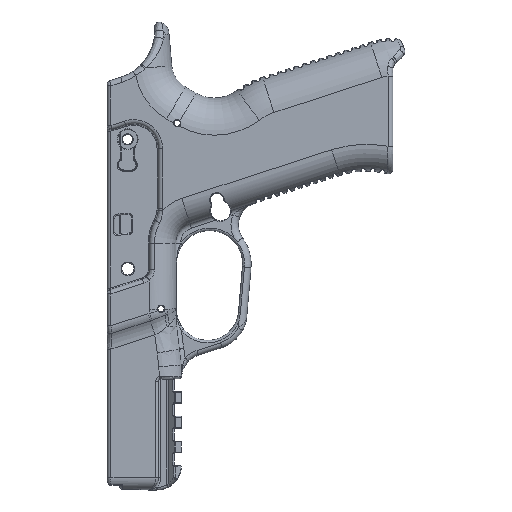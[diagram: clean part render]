
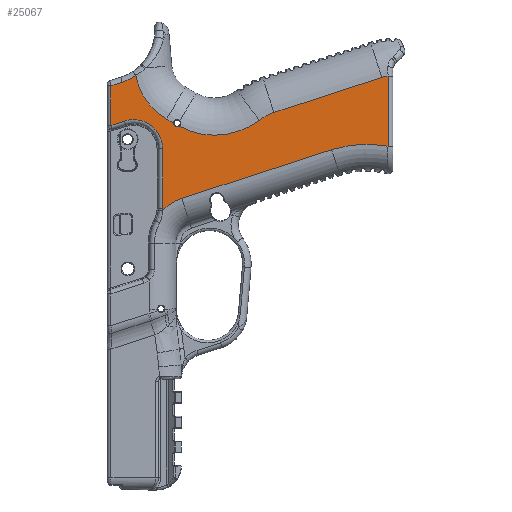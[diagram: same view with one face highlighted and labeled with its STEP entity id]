
A CAD part, left-side view. The second image highlights one B-rep face of the part: STEP entity #25067.
In plain terms, the highlighted planar face has unit normal (-1, 0, 0).
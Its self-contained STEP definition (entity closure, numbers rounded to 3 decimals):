
#246=PLANE('',#27413);
#535=LINE('',#38847,#1671);
#678=LINE('',#45280,#1814);
#984=LINE('',#53656,#2120);
#985=LINE('',#53662,#2121);
#986=LINE('',#53664,#2122);
#987=LINE('',#53666,#2123);
#988=LINE('',#53670,#2124);
#989=LINE('',#53675,#2125);
#1671=VECTOR('',#29705,10.);
#1814=VECTOR('',#30608,10.);
#2120=VECTOR('',#32378,10.);
#2121=VECTOR('',#32383,10.);
#2122=VECTOR('',#32384,10.);
#2123=VECTOR('',#32385,10.);
#2124=VECTOR('',#32388,10.);
#2125=VECTOR('',#32393,10.);
#4097=FACE_OUTER_BOUND('',#5734,.T.);
#5734=EDGE_LOOP('',(#19691,#19692,#19693,#19694,#19695,#19696,#19697,#19698,
#19699,#19700,#19701,#19702,#19703,#19704,#19705,#19706,#19707,#19708,#19709,
#19710));
#7162=CIRCLE('',#26238,20.);
#7449=CIRCLE('',#26915,46.);
#7712=CIRCLE('',#27407,1.44);
#7714=CIRCLE('',#27410,30.);
#7717=CIRCLE('',#27414,26.);
#7718=CIRCLE('',#27415,22.);
#7719=CIRCLE('',#27416,11.75);
#7720=CIRCLE('',#27417,11.75);
#7721=CIRCLE('',#27418,19.);
#7722=CIRCLE('',#27419,13.);
#9006=B_SPLINE_CURVE_WITH_KNOTS('',3,(#53617,#53618,#53619,#53620),
 .UNSPECIFIED.,.F.,.F.,(4,4),(0.244,0.253),
 .UNSPECIFIED.);
#9008=B_SPLINE_CURVE_WITH_KNOTS('',3,(#53641,#53642,#53643,#53644),
 .UNSPECIFIED.,.F.,.F.,(4,4),(0.052,0.062),
 .UNSPECIFIED.);
#9708=VERTEX_POINT('',#37754);
#9709=VERTEX_POINT('',#37756);
#9775=VERTEX_POINT('',#38846);
#10185=VERTEX_POINT('',#45277);
#10186=VERTEX_POINT('',#45279);
#10414=VERTEX_POINT('',#49002);
#10813=VERTEX_POINT('',#53458);
#10817=VERTEX_POINT('',#53496);
#10818=VERTEX_POINT('',#53498);
#10820=VERTEX_POINT('',#53563);
#10824=VERTEX_POINT('',#53655);
#10825=VERTEX_POINT('',#53657);
#10826=VERTEX_POINT('',#53659);
#10827=VERTEX_POINT('',#53661);
#10828=VERTEX_POINT('',#53663);
#10829=VERTEX_POINT('',#53665);
#10830=VERTEX_POINT('',#53667);
#10831=VERTEX_POINT('',#53669);
#10832=VERTEX_POINT('',#53671);
#10833=VERTEX_POINT('',#53674);
#12171=EDGE_CURVE('',#9708,#9709,#7162,.T.);
#12275=EDGE_CURVE('',#9709,#9775,#535,.T.);
#12896=EDGE_CURVE('',#10185,#10186,#678,.T.);
#13259=EDGE_CURVE('',#10414,#10185,#7449,.T.);
#13918=EDGE_CURVE('',#10817,#10818,#7712,.T.);
#13925=EDGE_CURVE('',#10820,#10817,#9006,.T.);
#13927=EDGE_CURVE('',#10818,#10813,#9008,.T.);
#13929=EDGE_CURVE('',#10813,#9708,#7714,.T.);
#13932=EDGE_CURVE('',#10824,#10820,#984,.T.);
#13933=EDGE_CURVE('',#10825,#10824,#7717,.T.);
#13934=EDGE_CURVE('',#10826,#10825,#7718,.T.);
#13935=EDGE_CURVE('',#10827,#10826,#985,.T.);
#13936=EDGE_CURVE('',#10828,#10827,#986,.T.);
#13937=EDGE_CURVE('',#10829,#10828,#987,.T.);
#13938=EDGE_CURVE('',#10830,#10829,#7719,.T.);
#13939=EDGE_CURVE('',#10831,#10830,#988,.T.);
#13940=EDGE_CURVE('',#10832,#10831,#7720,.T.);
#13941=EDGE_CURVE('',#10186,#10832,#7721,.T.);
#13942=EDGE_CURVE('',#10833,#10414,#989,.T.);
#13943=EDGE_CURVE('',#9775,#10833,#7722,.T.);
#19691=ORIENTED_EDGE('',*,*,#13927,.F.);
#19692=ORIENTED_EDGE('',*,*,#13918,.F.);
#19693=ORIENTED_EDGE('',*,*,#13925,.F.);
#19694=ORIENTED_EDGE('',*,*,#13932,.F.);
#19695=ORIENTED_EDGE('',*,*,#13933,.F.);
#19696=ORIENTED_EDGE('',*,*,#13934,.F.);
#19697=ORIENTED_EDGE('',*,*,#13935,.F.);
#19698=ORIENTED_EDGE('',*,*,#13936,.F.);
#19699=ORIENTED_EDGE('',*,*,#13937,.F.);
#19700=ORIENTED_EDGE('',*,*,#13938,.F.);
#19701=ORIENTED_EDGE('',*,*,#13939,.F.);
#19702=ORIENTED_EDGE('',*,*,#13940,.F.);
#19703=ORIENTED_EDGE('',*,*,#13941,.F.);
#19704=ORIENTED_EDGE('',*,*,#12896,.F.);
#19705=ORIENTED_EDGE('',*,*,#13259,.F.);
#19706=ORIENTED_EDGE('',*,*,#13942,.F.);
#19707=ORIENTED_EDGE('',*,*,#13943,.F.);
#19708=ORIENTED_EDGE('',*,*,#12275,.F.);
#19709=ORIENTED_EDGE('',*,*,#12171,.F.);
#19710=ORIENTED_EDGE('',*,*,#13929,.F.);
#25067=ADVANCED_FACE('',(#4097),#246,.F.);
#26238=AXIS2_PLACEMENT_3D('',#37757,#29557,#29558);
#26915=AXIS2_PLACEMENT_3D('',#49010,#31153,#31154);
#27407=AXIS2_PLACEMENT_3D('',#53499,#32362,#32363);
#27410=AXIS2_PLACEMENT_3D('',#53650,#32370,#32371);
#27413=AXIS2_PLACEMENT_3D('',#53654,#32376,#32377);
#27414=AXIS2_PLACEMENT_3D('',#53658,#32379,#32380);
#27415=AXIS2_PLACEMENT_3D('',#53660,#32381,#32382);
#27416=AXIS2_PLACEMENT_3D('',#53668,#32386,#32387);
#27417=AXIS2_PLACEMENT_3D('',#53672,#32389,#32390);
#27418=AXIS2_PLACEMENT_3D('',#53673,#32391,#32392);
#27419=AXIS2_PLACEMENT_3D('',#53676,#32394,#32395);
#29557=DIRECTION('center_axis',(1.,0.,0.));
#29558=DIRECTION('ref_axis',(0.,0.463,0.886));
#29705=DIRECTION('',(0.,-0.951,0.309));
#30608=DIRECTION('',(0.,0.951,-0.309));
#31153=DIRECTION('center_axis',(-1.,0.,0.));
#31154=DIRECTION('ref_axis',(0.,-0.012,1.));
#32362=DIRECTION('center_axis',(-1.,0.,0.));
#32363=DIRECTION('ref_axis',(0.,0.,-1.));
#32370=DIRECTION('center_axis',(-1.,0.,0.));
#32371=DIRECTION('ref_axis',(0.,-0.062,-0.998));
#32376=DIRECTION('center_axis',(1.,0.,0.));
#32377=DIRECTION('ref_axis',(0.,0.,-1.));
#32378=DIRECTION('',(0.,-0.866,-0.5));
#32379=DIRECTION('center_axis',(-1.,0.,0.));
#32380=DIRECTION('ref_axis',(0.,0.843,-0.537));
#32381=DIRECTION('center_axis',(-1.,0.,0.));
#32382=DIRECTION('ref_axis',(0.,-0.459,-0.889));
#32383=DIRECTION('',(0.,-0.951,0.309));
#32384=DIRECTION('',(0.,0.,1.));
#32385=DIRECTION('',(0.,0.951,-0.309));
#32386=DIRECTION('center_axis',(-1.,0.,0.));
#32387=DIRECTION('ref_axis',(0.,-0.588,0.809));
#32388=DIRECTION('',(0.,0.,1.));
#32389=DIRECTION('center_axis',(-1.,0.,0.));
#32390=DIRECTION('ref_axis',(0.,-0.968,-0.25));
#32391=DIRECTION('center_axis',(-1.,0.,0.));
#32392=DIRECTION('ref_axis',(0.,0.809,0.588));
#32393=DIRECTION('',(0.,0.,-1.));
#32394=DIRECTION('center_axis',(1.,0.,0.));
#32395=DIRECTION('ref_axis',(0.,0.129,0.992));
#37754=CARTESIAN_POINT('',(-16.,-8.989,66.499));
#37756=CARTESIAN_POINT('',(-16.,-14.885,69.578));
#37757=CARTESIAN_POINT('Origin',(-16.,-21.066,50.557));
#38846=CARTESIAN_POINT('',(-16.,-58.483,83.744));
#38847=CARTESIAN_POINT('',(-16.,-1.581,65.256));
#45277=CARTESIAN_POINT('',(-16.,-38.199,54.547));
#45279=CARTESIAN_POINT('',(-16.,22.371,34.867));
#45280=CARTESIAN_POINT('',(-16.,-16.559,47.516));
#49002=CARTESIAN_POINT('',(-16.,-61.,55.99));
#49010=CARTESIAN_POINT('Origin',(-16.,-52.414,10.798));
#53458=CARTESIAN_POINT('',(-16.,23.443,64.048));
#53496=CARTESIAN_POINT('',(-16.,25.69,65.222));
#53498=CARTESIAN_POINT('',(-16.,23.54,63.988));
#53499=CARTESIAN_POINT('Origin',(-16.,24.25,65.241));
#53563=CARTESIAN_POINT('',(-16.,25.687,65.332));
#53617=CARTESIAN_POINT('Ctrl Pts',(-16.,25.687,65.332));
#53618=CARTESIAN_POINT('Ctrl Pts',(-16.,25.689,65.295));
#53619=CARTESIAN_POINT('Ctrl Pts',(-16.,25.69,65.258));
#53620=CARTESIAN_POINT('Ctrl Pts',(-16.,25.69,65.222));
#53641=CARTESIAN_POINT('Ctrl Pts',(-16.,23.54,63.988));
#53642=CARTESIAN_POINT('Ctrl Pts',(-16.,23.507,64.007));
#53643=CARTESIAN_POINT('Ctrl Pts',(-16.,23.474,64.027));
#53644=CARTESIAN_POINT('Ctrl Pts',(-16.,23.443,64.048));
#53650=CARTESIAN_POINT('Origin',(-16.,9.127,90.412));
#53654=CARTESIAN_POINT('Origin',(-16.,-7.789,0.877));
#53655=CARTESIAN_POINT('',(-16.,28.457,66.931));
#53656=CARTESIAN_POINT('',(-16.,0.564,50.827));
#53657=CARTESIAN_POINT('',(-16.,40.986,84.52));
#53658=CARTESIAN_POINT('Origin',(-16.,15.457,89.448));
#53659=CARTESIAN_POINT('',(-16.,46.448,81.863));
#53660=CARTESIAN_POINT('Origin',(-16.,53.246,102.787));
#53661=CARTESIAN_POINT('',(-16.,51.,80.384));
#53662=CARTESIAN_POINT('',(-16.,36.537,85.084));
#53663=CARTESIAN_POINT('',(-16.,51.,64.35));
#53664=CARTESIAN_POINT('',(-16.,51.,-51.061));
#53665=CARTESIAN_POINT('',(-16.,45.502,66.136));
#53666=CARTESIAN_POINT('',(-16.,34.76,69.626));
#53667=CARTESIAN_POINT('',(-16.,30.121,54.961));
#53668=CARTESIAN_POINT('Origin',(-16.,41.871,54.961));
#53669=CARTESIAN_POINT('',(-16.,30.121,30.843));
#53670=CARTESIAN_POINT('',(-16.,30.121,27.919));
#53671=CARTESIAN_POINT('',(-16.,30.151,30.012));
#53672=CARTESIAN_POINT('Origin',(-16.,41.871,30.843));
#53673=CARTESIAN_POINT('Origin',(-16.,16.5,16.797));
#53674=CARTESIAN_POINT('',(-16.,-61.,84.294));
#53675=CARTESIAN_POINT('',(-16.,-61.,44.851));
#53676=CARTESIAN_POINT('Origin',(-16.,-62.5,71.38));
